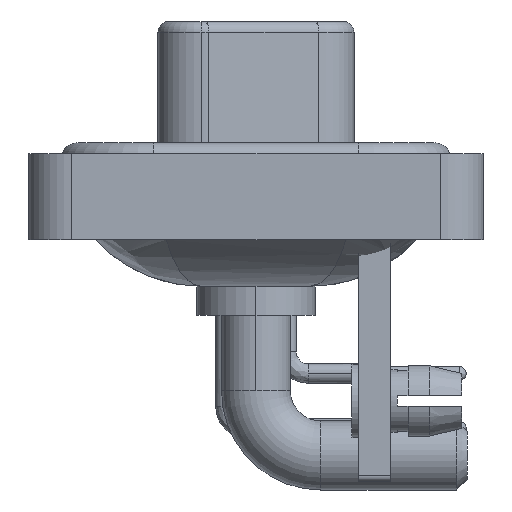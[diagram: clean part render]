
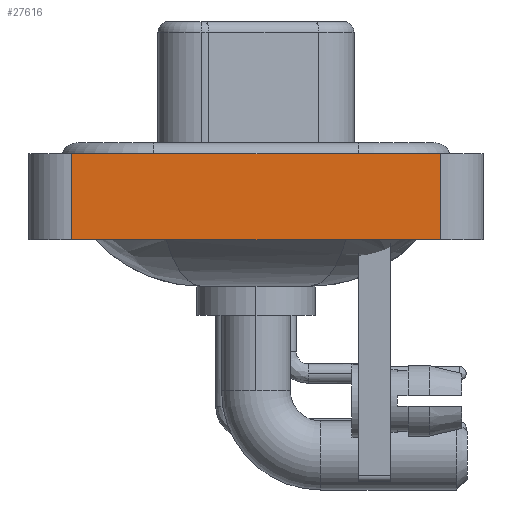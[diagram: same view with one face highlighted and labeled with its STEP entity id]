
A CAD part, left-side view. The second image highlights one B-rep face of the part: STEP entity #27616.
In plain terms, the highlighted planar face has unit normal (-1, 0, 0).
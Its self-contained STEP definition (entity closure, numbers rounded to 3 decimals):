
#422 = VECTOR ( 'NONE', #21530, 1000. ) ;
#471 = LINE ( 'NONE', #24155, #6011 ) ;
#521 = LINE ( 'NONE', #16866, #422 ) ;
#1270 = DIRECTION ( 'NONE',  ( -1., 0., 0. ) ) ;
#1987 = CARTESIAN_POINT ( 'NONE',  ( -7.35, -8.55, -3.6 ) ) ;
#2017 = EDGE_CURVE ( 'NONE', #5123, #18858, #521, .T. ) ;
#2880 = EDGE_LOOP ( 'NONE', ( #5646, #10763, #13143, #4016 ) ) ;
#3440 = PLANE ( 'NONE',  #30001 ) ;
#4016 = ORIENTED_EDGE ( 'NONE', *, *, #16795, .T. ) ;
#4478 = EDGE_CURVE ( 'NONE', #18345, #5123, #471, .T. ) ;
#5123 = VERTEX_POINT ( 'NONE', #13775 ) ;
#5646 = ORIENTED_EDGE ( 'NONE', *, *, #24904, .T. ) ;
#6011 = VECTOR ( 'NONE', #12267, 1000. ) ;
#7148 = CARTESIAN_POINT ( 'NONE',  ( -7.35, -8.55, 0.4 ) ) ;
#10763 = ORIENTED_EDGE ( 'NONE', *, *, #2017, .F. ) ;
#11158 = LINE ( 'NONE', #1987, #14288 ) ;
#11479 = CARTESIAN_POINT ( 'NONE',  ( -7.35, -8.55, -3.6 ) ) ;
#12267 = DIRECTION ( 'NONE',  ( 0., 0., 1. ) ) ;
#13143 = ORIENTED_EDGE ( 'NONE', *, *, #4478, .F. ) ;
#13775 = CARTESIAN_POINT ( 'NONE',  ( -7.35, 8.55, 0.4 ) ) ;
#14288 = VECTOR ( 'NONE', #20968, 1000. ) ;
#16224 = CARTESIAN_POINT ( 'NONE',  ( -7.35, 8.55, -3.6 ) ) ;
#16470 = DIRECTION ( 'NONE',  ( 0., -1., 0. ) ) ;
#16795 = EDGE_CURVE ( 'NONE', #18345, #24945, #18661, .T. ) ;
#16866 = CARTESIAN_POINT ( 'NONE',  ( -7.35, -8.55, 0.4 ) ) ;
#18345 = VERTEX_POINT ( 'NONE', #16224 ) ;
#18661 = LINE ( 'NONE', #11479, #23130 ) ;
#18858 = VERTEX_POINT ( 'NONE', #7148 ) ;
#19942 = CARTESIAN_POINT ( 'NONE',  ( -7.35, -8.55, -3.6 ) ) ;
#20091 = FACE_OUTER_BOUND ( 'NONE', #2880, .T. ) ;
#20968 = DIRECTION ( 'NONE',  ( 0., 0., 1. ) ) ;
#21530 = DIRECTION ( 'NONE',  ( 0., -1., 0. ) ) ;
#23130 = VECTOR ( 'NONE', #16470, 1000. ) ;
#23795 = CARTESIAN_POINT ( 'NONE',  ( -7.35, -8.55, -3.6 ) ) ;
#24155 = CARTESIAN_POINT ( 'NONE',  ( -7.35, 8.55, -3.6 ) ) ;
#24904 = EDGE_CURVE ( 'NONE', #24945, #18858, #11158, .T. ) ;
#24945 = VERTEX_POINT ( 'NONE', #23795 ) ;
#27616 = ADVANCED_FACE ( 'NONE', ( #20091 ), #3440, .T. ) ;
#29789 = DIRECTION ( 'NONE',  ( 0., 0., 1. ) ) ;
#30001 = AXIS2_PLACEMENT_3D ( 'NONE', #19942, #1270, #29789 ) ;
